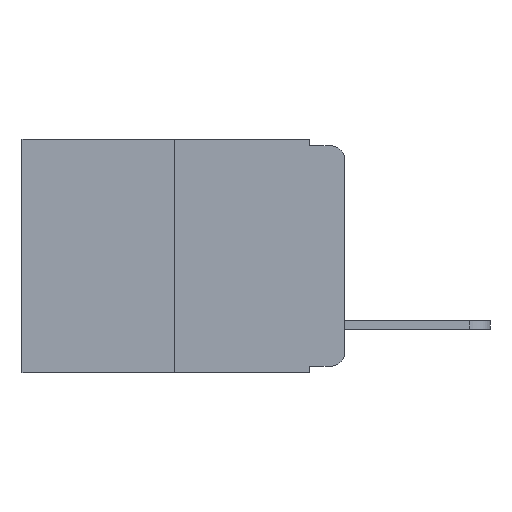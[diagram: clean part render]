
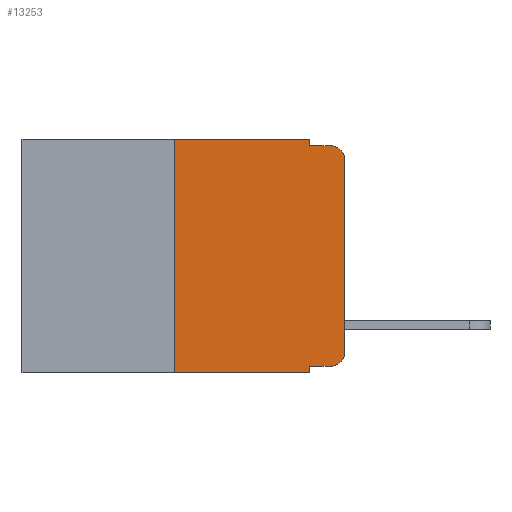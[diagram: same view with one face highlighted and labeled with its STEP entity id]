
A CAD part, left-side view. The second image highlights one B-rep face of the part: STEP entity #13253.
In plain terms, the highlighted planar face has unit normal (-1, 0, 0).
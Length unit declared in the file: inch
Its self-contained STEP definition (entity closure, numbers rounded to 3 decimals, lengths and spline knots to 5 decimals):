
#90 = EDGE_CURVE ( 'NONE', #16395, #9125, #8703, .T. ) ;
#294 = DIRECTION ( 'NONE',  ( 0., 0., -1. ) ) ;
#480 = LINE ( 'NONE', #11317, #10112 ) ;
#557 = ORIENTED_EDGE ( 'NONE', *, *, #15778, .T. ) ;
#796 = LINE ( 'NONE', #21714, #19076 ) ;
#859 = EDGE_CURVE ( 'NONE', #12058, #5996, #480, .T. ) ;
#1131 = ORIENTED_EDGE ( 'NONE', *, *, #10790, .F. ) ;
#1817 = DIRECTION ( 'NONE',  ( 0., -1., 0. ) ) ;
#2011 = VERTEX_POINT ( 'NONE', #19397 ) ;
#2126 = CARTESIAN_POINT ( 'NONE',  ( 0., 0.051, 0. ) ) ;
#2130 = DIRECTION ( 'NONE',  ( 0., 0., -1. ) ) ;
#2379 = VECTOR ( 'NONE', #1817, 39.37008 ) ;
#2911 = DIRECTION ( 'NONE',  ( 0., 0., 1. ) ) ;
#3078 = CARTESIAN_POINT ( 'NONE',  ( 0., 0.25, 0. ) ) ;
#3225 = CARTESIAN_POINT ( 'NONE',  ( 0., 0.051, -0.343 ) ) ;
#3478 = VERTEX_POINT ( 'NONE', #13991 ) ;
#3679 = VECTOR ( 'NONE', #21987, 39.37008 ) ;
#4482 = AXIS2_PLACEMENT_3D ( 'NONE', #20339, #9213, #22048 ) ;
#5611 = CARTESIAN_POINT ( 'NONE',  ( 0., 0.051, -0.01 ) ) ;
#5996 = VERTEX_POINT ( 'NONE', #3225 ) ;
#6403 = LINE ( 'NONE', #2126, #15793 ) ;
#7221 = ORIENTED_EDGE ( 'NONE', *, *, #14553, .F. ) ;
#7388 = LINE ( 'NONE', #19994, #17275 ) ;
#7844 = CARTESIAN_POINT ( 'NONE',  ( 0., 0.02, -0.333 ) ) ;
#8084 = AXIS2_PLACEMENT_3D ( 'NONE', #22639, #11827, #294 ) ;
#8187 = AXIS2_PLACEMENT_3D ( 'NONE', #23541, #23204, #23175 ) ;
#8252 = EDGE_CURVE ( 'NONE', #16395, #5996, #796, .T. ) ;
#8703 = LINE ( 'NONE', #10161, #3679 ) ;
#8851 = VERTEX_POINT ( 'NONE', #13076 ) ;
#9125 = VERTEX_POINT ( 'NONE', #7844 ) ;
#9213 = DIRECTION ( 'NONE',  ( -1., 0., 0. ) ) ;
#9310 = ORIENTED_EDGE ( 'NONE', *, *, #90, .T. ) ;
#9813 = ORIENTED_EDGE ( 'NONE', *, *, #12729, .F. ) ;
#10112 = VECTOR ( 'NONE', #21863, 39.37008 ) ;
#10161 = CARTESIAN_POINT ( 'NONE',  ( 0., 0.051, -0.333 ) ) ;
#10192 = CARTESIAN_POINT ( 'NONE',  ( 0., 0.25, -0.343 ) ) ;
#10535 = EDGE_LOOP ( 'NONE', ( #22215, #557, #12842, #7221, #9813, #1131, #23540, #23779, #9310, #10846 ) ) ;
#10790 = EDGE_CURVE ( 'NONE', #12058, #2011, #15764, .T. ) ;
#10815 = VECTOR ( 'NONE', #2911, 39.37008 ) ;
#10846 = ORIENTED_EDGE ( 'NONE', *, *, #23022, .T. ) ;
#11317 = CARTESIAN_POINT ( 'NONE',  ( 0., 0.473, -0.343 ) ) ;
#11827 = DIRECTION ( 'NONE',  ( -1., 0., 0. ) ) ;
#12058 = VERTEX_POINT ( 'NONE', #10192 ) ;
#12433 = LINE ( 'NONE', #5611, #2379 ) ;
#12553 = VERTEX_POINT ( 'NONE', #23030 ) ;
#12729 = EDGE_CURVE ( 'NONE', #2011, #19768, #19617, .T. ) ;
#12842 = ORIENTED_EDGE ( 'NONE', *, *, #17008, .F. ) ;
#13076 = CARTESIAN_POINT ( 'NONE',  ( 0., 0., -0.03 ) ) ;
#13253 = ADVANCED_FACE ( 'NONE', ( #21022 ), #23242, .F. ) ;
#13991 = CARTESIAN_POINT ( 'NONE',  ( 0., 0.051, -0.01 ) ) ;
#14226 = CARTESIAN_POINT ( 'NONE',  ( 0., 0., -0.313 ) ) ;
#14553 = EDGE_CURVE ( 'NONE', #19768, #3478, #6403, .T. ) ;
#14801 = VECTOR ( 'NONE', #17867, 39.37008 ) ;
#15269 = VERTEX_POINT ( 'NONE', #14226 ) ;
#15764 = LINE ( 'NONE', #3078, #10815 ) ;
#15778 = EDGE_CURVE ( 'NONE', #8851, #12553, #16563, .T. ) ;
#15793 = VECTOR ( 'NONE', #2130, 39.37008 ) ;
#16395 = VERTEX_POINT ( 'NONE', #22413 ) ;
#16563 = CIRCLE ( 'NONE', #8084, 0.02 ) ;
#17008 = EDGE_CURVE ( 'NONE', #3478, #12553, #12433, .T. ) ;
#17093 = CIRCLE ( 'NONE', #4482, 0.02 ) ;
#17275 = VECTOR ( 'NONE', #21729, 39.37008 ) ;
#17867 = DIRECTION ( 'NONE',  ( 0., -1., 0. ) ) ;
#18771 = CARTESIAN_POINT ( 'NONE',  ( 0., 0.473, 0. ) ) ;
#18937 = CARTESIAN_POINT ( 'NONE',  ( 0., 0.051, 0. ) ) ;
#19076 = VECTOR ( 'NONE', #21643, 39.37008 ) ;
#19397 = CARTESIAN_POINT ( 'NONE',  ( 0., 0.25, 0. ) ) ;
#19422 = EDGE_CURVE ( 'NONE', #15269, #8851, #7388, .T. ) ;
#19617 = LINE ( 'NONE', #18771, #14801 ) ;
#19768 = VERTEX_POINT ( 'NONE', #18937 ) ;
#19994 = CARTESIAN_POINT ( 'NONE',  ( 0., 0., 0. ) ) ;
#20339 = CARTESIAN_POINT ( 'NONE',  ( 0., 0.02, -0.313 ) ) ;
#21022 = FACE_OUTER_BOUND ( 'NONE', #10535, .T. ) ;
#21643 = DIRECTION ( 'NONE',  ( 0., 0., -1. ) ) ;
#21714 = CARTESIAN_POINT ( 'NONE',  ( 0., 0.051, 0. ) ) ;
#21729 = DIRECTION ( 'NONE',  ( 0., 0., 1. ) ) ;
#21863 = DIRECTION ( 'NONE',  ( 0., -1., 0. ) ) ;
#21987 = DIRECTION ( 'NONE',  ( 0., -1., 0. ) ) ;
#22048 = DIRECTION ( 'NONE',  ( 0., 0., -1. ) ) ;
#22215 = ORIENTED_EDGE ( 'NONE', *, *, #19422, .T. ) ;
#22413 = CARTESIAN_POINT ( 'NONE',  ( 0., 0.051, -0.333 ) ) ;
#22639 = CARTESIAN_POINT ( 'NONE',  ( 0., 0.02, -0.03 ) ) ;
#23022 = EDGE_CURVE ( 'NONE', #9125, #15269, #17093, .T. ) ;
#23030 = CARTESIAN_POINT ( 'NONE',  ( 0., 0.02, -0.01 ) ) ;
#23175 = DIRECTION ( 'NONE',  ( 0., 0., -1. ) ) ;
#23204 = DIRECTION ( 'NONE',  ( 1., 0., 0. ) ) ;
#23242 = PLANE ( 'NONE',  #8187 ) ;
#23540 = ORIENTED_EDGE ( 'NONE', *, *, #859, .T. ) ;
#23541 = CARTESIAN_POINT ( 'NONE',  ( 0., 0.473, 0. ) ) ;
#23779 = ORIENTED_EDGE ( 'NONE', *, *, #8252, .F. ) ;
